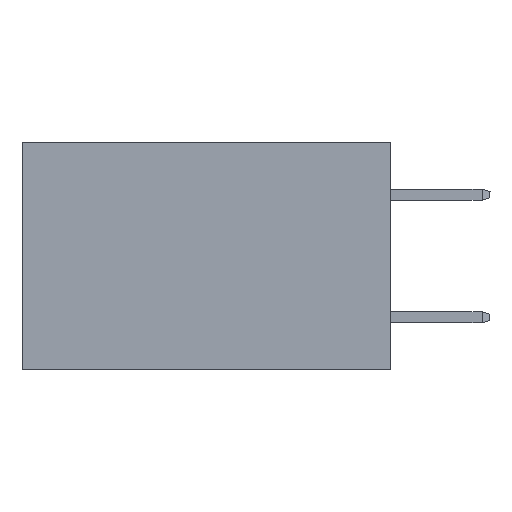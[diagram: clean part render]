
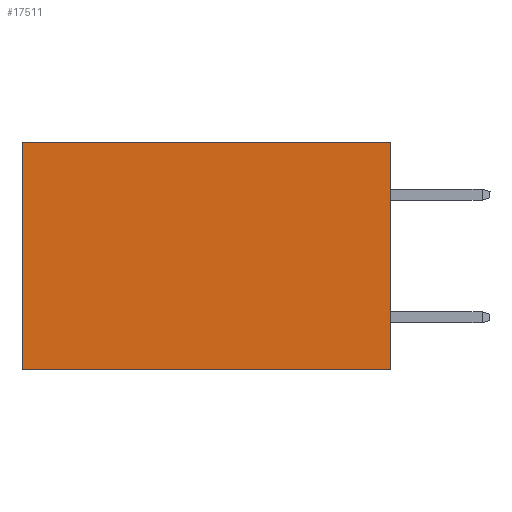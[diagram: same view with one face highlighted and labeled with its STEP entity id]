
A CAD part, left-side view. The second image highlights one B-rep face of the part: STEP entity #17511.
In plain terms, the highlighted planar face has unit normal (-1, 0, 0).
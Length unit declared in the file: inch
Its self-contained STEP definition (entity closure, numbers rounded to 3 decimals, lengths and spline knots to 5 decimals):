
#781 = CARTESIAN_POINT ( 'NONE',  ( 0.2875, 0., 0. ) ) ;
#1208 = VECTOR ( 'NONE', #19811, 39.37008 ) ;
#1534 = CARTESIAN_POINT ( 'NONE',  ( 0.2875, 0.6, 0. ) ) ;
#4657 = DIRECTION ( 'NONE',  ( 1., 0., 0. ) ) ;
#5699 = EDGE_CURVE ( 'NONE', #9090, #23268, #14602, .T. ) ;
#6336 = PLANE ( 'NONE',  #10530 ) ;
#6625 = EDGE_CURVE ( 'NONE', #23268, #6939, #12629, .T. ) ;
#6939 = VERTEX_POINT ( 'NONE', #10733 ) ;
#7070 = CARTESIAN_POINT ( 'NONE',  ( 0.2875, 0., 0. ) ) ;
#7290 = LINE ( 'NONE', #16694, #14921 ) ;
#7946 = FACE_OUTER_BOUND ( 'NONE', #16463, .T. ) ;
#9090 = VERTEX_POINT ( 'NONE', #21713 ) ;
#9741 = CARTESIAN_POINT ( 'NONE',  ( 0.2875, 0.6, 0. ) ) ;
#9992 = ORIENTED_EDGE ( 'NONE', *, *, #13784, .F. ) ;
#10530 = AXIS2_PLACEMENT_3D ( 'NONE', #781, #4657, #17401 ) ;
#10733 = CARTESIAN_POINT ( 'NONE',  ( 0.2875, 0.6, -0.37 ) ) ;
#11802 = EDGE_CURVE ( 'NONE', #9090, #13386, #7290, .T. ) ;
#12629 = LINE ( 'NONE', #1534, #13198 ) ;
#12718 = ORIENTED_EDGE ( 'NONE', *, *, #11802, .F. ) ;
#12937 = VECTOR ( 'NONE', #22703, 39.37008 ) ;
#13174 = CARTESIAN_POINT ( 'NONE',  ( 0.2875, 0., -0.37 ) ) ;
#13198 = VECTOR ( 'NONE', #16656, 39.37008 ) ;
#13386 = VERTEX_POINT ( 'NONE', #13174 ) ;
#13538 = ORIENTED_EDGE ( 'NONE', *, *, #5699, .T. ) ;
#13784 = EDGE_CURVE ( 'NONE', #13386, #6939, #23540, .T. ) ;
#14602 = LINE ( 'NONE', #7070, #1208 ) ;
#14921 = VECTOR ( 'NONE', #18386, 39.37008 ) ;
#15409 = CARTESIAN_POINT ( 'NONE',  ( 0.2875, 0., -0.37 ) ) ;
#16463 = EDGE_LOOP ( 'NONE', ( #17049, #9992, #12718, #13538 ) ) ;
#16656 = DIRECTION ( 'NONE',  ( 0., 0., -1. ) ) ;
#16694 = CARTESIAN_POINT ( 'NONE',  ( 0.2875, 0., 0. ) ) ;
#17049 = ORIENTED_EDGE ( 'NONE', *, *, #6625, .T. ) ;
#17401 = DIRECTION ( 'NONE',  ( 0., 0., -1. ) ) ;
#17511 = ADVANCED_FACE ( 'NONE', ( #7946 ), #6336, .F. ) ;
#18386 = DIRECTION ( 'NONE',  ( 0., 0., -1. ) ) ;
#19811 = DIRECTION ( 'NONE',  ( 0., 1., 0. ) ) ;
#21713 = CARTESIAN_POINT ( 'NONE',  ( 0.2875, 0., 0. ) ) ;
#22703 = DIRECTION ( 'NONE',  ( 0., 1., 0. ) ) ;
#23268 = VERTEX_POINT ( 'NONE', #9741 ) ;
#23540 = LINE ( 'NONE', #15409, #12937 ) ;
